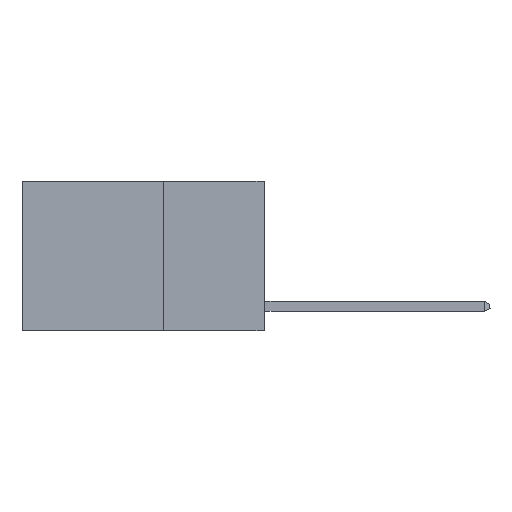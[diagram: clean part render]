
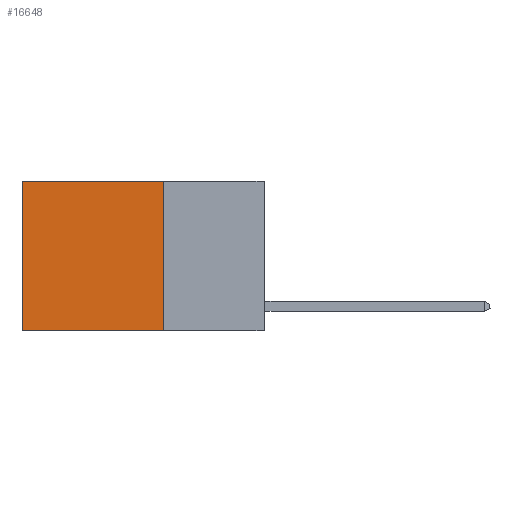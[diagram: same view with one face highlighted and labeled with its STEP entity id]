
A CAD part, left-side view. The second image highlights one B-rep face of the part: STEP entity #16648.
In plain terms, the highlighted planar face has unit normal (-1, 0, 0).
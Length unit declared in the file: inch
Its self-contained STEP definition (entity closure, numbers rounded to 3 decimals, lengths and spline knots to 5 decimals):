
#576 = VECTOR ( 'NONE', #12550, 39.37008 ) ;
#734 = EDGE_CURVE ( 'NONE', #20065, #20743, #4929, .T. ) ;
#749 = DIRECTION ( 'NONE',  ( 0., 0., -1. ) ) ;
#2243 = LINE ( 'NONE', #16498, #8546 ) ;
#2404 = CARTESIAN_POINT ( 'NONE',  ( 0.2625, 0.6, 0. ) ) ;
#3338 = DIRECTION ( 'NONE',  ( 0., 0., -1. ) ) ;
#3768 = CARTESIAN_POINT ( 'NONE',  ( 0.2625, 0.25, 0. ) ) ;
#4537 = ORIENTED_EDGE ( 'NONE', *, *, #19938, .F. ) ;
#4929 = LINE ( 'NONE', #19172, #5531 ) ;
#5531 = VECTOR ( 'NONE', #749, 39.37008 ) ;
#5629 = CARTESIAN_POINT ( 'NONE',  ( 0.2625, 0.25, -0.37 ) ) ;
#5853 = CARTESIAN_POINT ( 'NONE',  ( 0.2625, 0.6, -0.37 ) ) ;
#8191 = CARTESIAN_POINT ( 'NONE',  ( 0.2625, 0.25, -0.37 ) ) ;
#8546 = VECTOR ( 'NONE', #22730, 39.37008 ) ;
#9158 = CARTESIAN_POINT ( 'NONE',  ( 0.2625, 0.25, 0. ) ) ;
#9965 = ORIENTED_EDGE ( 'NONE', *, *, #734, .T. ) ;
#10061 = VECTOR ( 'NONE', #12056, 39.37008 ) ;
#12056 = DIRECTION ( 'NONE',  ( 0., 0., -1. ) ) ;
#12440 = VERTEX_POINT ( 'NONE', #5629 ) ;
#12550 = DIRECTION ( 'NONE',  ( 0., 1., 0. ) ) ;
#15522 = EDGE_CURVE ( 'NONE', #12440, #20743, #20807, .T. ) ;
#15820 = PLANE ( 'NONE',  #17462 ) ;
#16498 = CARTESIAN_POINT ( 'NONE',  ( 0.2625, 0.25, 0. ) ) ;
#16648 = ADVANCED_FACE ( 'NONE', ( #21776 ), #15820, .F. ) ;
#17462 = AXIS2_PLACEMENT_3D ( 'NONE', #9158, #17729, #3338 ) ;
#17729 = DIRECTION ( 'NONE',  ( 1., 0., 0. ) ) ;
#19172 = CARTESIAN_POINT ( 'NONE',  ( 0.2625, 0.6, 0. ) ) ;
#19938 = EDGE_CURVE ( 'NONE', #26687, #12440, #20444, .T. ) ;
#20065 = VERTEX_POINT ( 'NONE', #2404 ) ;
#20301 = CARTESIAN_POINT ( 'NONE',  ( 0.2625, 0.25, 0. ) ) ;
#20444 = LINE ( 'NONE', #3768, #10061 ) ;
#20743 = VERTEX_POINT ( 'NONE', #5853 ) ;
#20807 = LINE ( 'NONE', #8191, #576 ) ;
#21352 = ORIENTED_EDGE ( 'NONE', *, *, #26572, .T. ) ;
#21776 = FACE_OUTER_BOUND ( 'NONE', #23462, .T. ) ;
#22730 = DIRECTION ( 'NONE',  ( 0., 1., 0. ) ) ;
#22945 = ORIENTED_EDGE ( 'NONE', *, *, #15522, .F. ) ;
#23462 = EDGE_LOOP ( 'NONE', ( #9965, #22945, #4537, #21352 ) ) ;
#26572 = EDGE_CURVE ( 'NONE', #26687, #20065, #2243, .T. ) ;
#26687 = VERTEX_POINT ( 'NONE', #20301 ) ;
